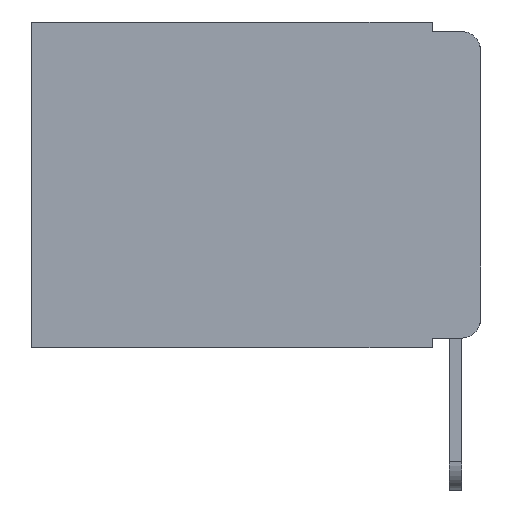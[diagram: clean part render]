
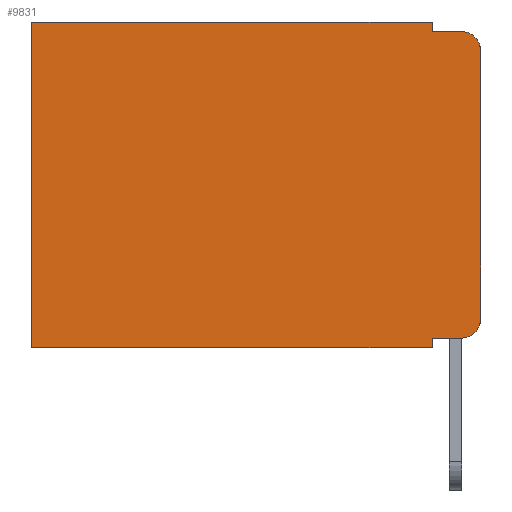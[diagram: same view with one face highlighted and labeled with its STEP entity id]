
A CAD part, left-side view. The second image highlights one B-rep face of the part: STEP entity #9831.
In plain terms, the highlighted planar face has unit normal (-1, 0, 0).
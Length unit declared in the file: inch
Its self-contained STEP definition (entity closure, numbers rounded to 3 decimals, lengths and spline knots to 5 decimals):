
#198 = CIRCLE ( 'NONE', #18089, 0.02 ) ;
#347 = DIRECTION ( 'NONE',  ( 0., 0., -1. ) ) ;
#386 = EDGE_CURVE ( 'NONE', #8803, #1927, #5893, .T. ) ;
#830 = DIRECTION ( 'NONE',  ( 0., 0., -1. ) ) ;
#938 = AXIS2_PLACEMENT_3D ( 'NONE', #8334, #9910, #347 ) ;
#1100 = VECTOR ( 'NONE', #18197, 39.37008 ) ;
#1686 = VERTEX_POINT ( 'NONE', #2902 ) ;
#1927 = VERTEX_POINT ( 'NONE', #13423 ) ;
#1942 = VECTOR ( 'NONE', #5613, 39.37008 ) ;
#2117 = VERTEX_POINT ( 'NONE', #18357 ) ;
#2232 = DIRECTION ( 'NONE',  ( 0., 1., 0. ) ) ;
#2385 = CARTESIAN_POINT ( 'NONE',  ( 0.298, 0., 0. ) ) ;
#2406 = LINE ( 'NONE', #14742, #13957 ) ;
#2709 = EDGE_LOOP ( 'NONE', ( #17388, #13794, #4979, #5236, #13564, #9372, #11828, #16150, #13344, #4747 ) ) ;
#2799 = CARTESIAN_POINT ( 'NONE',  ( 0.298, 0.473, 0. ) ) ;
#2902 = CARTESIAN_POINT ( 'NONE',  ( 0.298, 0.02, -0.01 ) ) ;
#3344 = DIRECTION ( 'NONE',  ( -1., 0., 0. ) ) ;
#4204 = LINE ( 'NONE', #12311, #18591 ) ;
#4363 = EDGE_CURVE ( 'NONE', #2117, #1686, #13730, .T. ) ;
#4403 = DIRECTION ( 'NONE',  ( 0., 0., -1. ) ) ;
#4747 = ORIENTED_EDGE ( 'NONE', *, *, #7667, .T. ) ;
#4826 = AXIS2_PLACEMENT_3D ( 'NONE', #12412, #3344, #13836 ) ;
#4979 = ORIENTED_EDGE ( 'NONE', *, *, #4363, .F. ) ;
#5184 = VERTEX_POINT ( 'NONE', #15734 ) ;
#5236 = ORIENTED_EDGE ( 'NONE', *, *, #7860, .F. ) ;
#5613 = DIRECTION ( 'NONE',  ( 0., 0., -1. ) ) ;
#5615 = CARTESIAN_POINT ( 'NONE',  ( 0.298, 0.473, -0.343 ) ) ;
#5893 = LINE ( 'NONE', #18171, #1100 ) ;
#5973 = CARTESIAN_POINT ( 'NONE',  ( 0.298, 0.051, -0.01 ) ) ;
#6446 = VERTEX_POINT ( 'NONE', #8741 ) ;
#6721 = EDGE_CURVE ( 'NONE', #5184, #11745, #4204, .T. ) ;
#6963 = EDGE_CURVE ( 'NONE', #12030, #15449, #10326, .T. ) ;
#7417 = EDGE_CURVE ( 'NONE', #6446, #13121, #15042, .T. ) ;
#7540 = EDGE_CURVE ( 'NONE', #11745, #13121, #17954, .T. ) ;
#7543 = EDGE_CURVE ( 'NONE', #8803, #6446, #2406, .T. ) ;
#7667 = EDGE_CURVE ( 'NONE', #1927, #15449, #14592, .T. ) ;
#7860 = EDGE_CURVE ( 'NONE', #5184, #2117, #15860, .T. ) ;
#8308 = VECTOR ( 'NONE', #830, 39.37008 ) ;
#8334 = CARTESIAN_POINT ( 'NONE',  ( 0.298, 0., 0. ) ) ;
#8371 = DIRECTION ( 'NONE',  ( -1., 0., 0. ) ) ;
#8741 = CARTESIAN_POINT ( 'NONE',  ( 0.298, 0.051, -0.343 ) ) ;
#8803 = VERTEX_POINT ( 'NONE', #18830 ) ;
#9372 = ORIENTED_EDGE ( 'NONE', *, *, #7540, .T. ) ;
#9534 = CARTESIAN_POINT ( 'NONE',  ( 0.298, 0., -0.313 ) ) ;
#9831 = ADVANCED_FACE ( 'NONE', ( #14381 ), #16767, .F. ) ;
#9910 = DIRECTION ( 'NONE',  ( 1., 0., 0. ) ) ;
#10007 = CARTESIAN_POINT ( 'NONE',  ( 0.298, 0., -0.03 ) ) ;
#10326 = LINE ( 'NONE', #2385, #1942 ) ;
#11549 = VECTOR ( 'NONE', #4403, 39.37008 ) ;
#11745 = VERTEX_POINT ( 'NONE', #13770 ) ;
#11828 = ORIENTED_EDGE ( 'NONE', *, *, #7417, .F. ) ;
#12030 = VERTEX_POINT ( 'NONE', #10007 ) ;
#12311 = CARTESIAN_POINT ( 'NONE',  ( 0.298, 0., 0. ) ) ;
#12412 = CARTESIAN_POINT ( 'NONE',  ( 0.298, 0.02, -0.313 ) ) ;
#13000 = CARTESIAN_POINT ( 'NONE',  ( 0.298, 0.051, 0. ) ) ;
#13121 = VERTEX_POINT ( 'NONE', #5615 ) ;
#13344 = ORIENTED_EDGE ( 'NONE', *, *, #386, .T. ) ;
#13423 = CARTESIAN_POINT ( 'NONE',  ( 0.298, 0.02, -0.333 ) ) ;
#13564 = ORIENTED_EDGE ( 'NONE', *, *, #6721, .T. ) ;
#13730 = LINE ( 'NONE', #5973, #17330 ) ;
#13770 = CARTESIAN_POINT ( 'NONE',  ( 0.298, 0.473, 0. ) ) ;
#13794 = ORIENTED_EDGE ( 'NONE', *, *, #15596, .T. ) ;
#13836 = DIRECTION ( 'NONE',  ( 0., 0., -1. ) ) ;
#13957 = VECTOR ( 'NONE', #16109, 39.37008 ) ;
#14381 = FACE_OUTER_BOUND ( 'NONE', #2709, .T. ) ;
#14592 = CIRCLE ( 'NONE', #4826, 0.02 ) ;
#14742 = CARTESIAN_POINT ( 'NONE',  ( 0.298, 0.051, 0. ) ) ;
#15042 = LINE ( 'NONE', #15670, #17758 ) ;
#15449 = VERTEX_POINT ( 'NONE', #9534 ) ;
#15596 = EDGE_CURVE ( 'NONE', #12030, #1686, #198, .T. ) ;
#15670 = CARTESIAN_POINT ( 'NONE',  ( 0.298, 0., -0.343 ) ) ;
#15734 = CARTESIAN_POINT ( 'NONE',  ( 0.298, 0.051, 0. ) ) ;
#15860 = LINE ( 'NONE', #13000, #8308 ) ;
#16109 = DIRECTION ( 'NONE',  ( 0., 0., -1. ) ) ;
#16150 = ORIENTED_EDGE ( 'NONE', *, *, #7543, .F. ) ;
#16485 = DIRECTION ( 'NONE',  ( 0., 1., 0. ) ) ;
#16767 = PLANE ( 'NONE',  #938 ) ;
#16797 = CARTESIAN_POINT ( 'NONE',  ( 0.298, 0.02, -0.03 ) ) ;
#16895 = DIRECTION ( 'NONE',  ( 0., -1., 0. ) ) ;
#17330 = VECTOR ( 'NONE', #16895, 39.37008 ) ;
#17388 = ORIENTED_EDGE ( 'NONE', *, *, #6963, .F. ) ;
#17758 = VECTOR ( 'NONE', #2232, 39.37008 ) ;
#17954 = LINE ( 'NONE', #2799, #11549 ) ;
#18089 = AXIS2_PLACEMENT_3D ( 'NONE', #16797, #8371, #18125 ) ;
#18125 = DIRECTION ( 'NONE',  ( 0., 0., -1. ) ) ;
#18171 = CARTESIAN_POINT ( 'NONE',  ( 0.298, 0.051, -0.333 ) ) ;
#18197 = DIRECTION ( 'NONE',  ( 0., -1., 0. ) ) ;
#18357 = CARTESIAN_POINT ( 'NONE',  ( 0.298, 0.051, -0.01 ) ) ;
#18591 = VECTOR ( 'NONE', #16485, 39.37008 ) ;
#18830 = CARTESIAN_POINT ( 'NONE',  ( 0.298, 0.051, -0.333 ) ) ;
